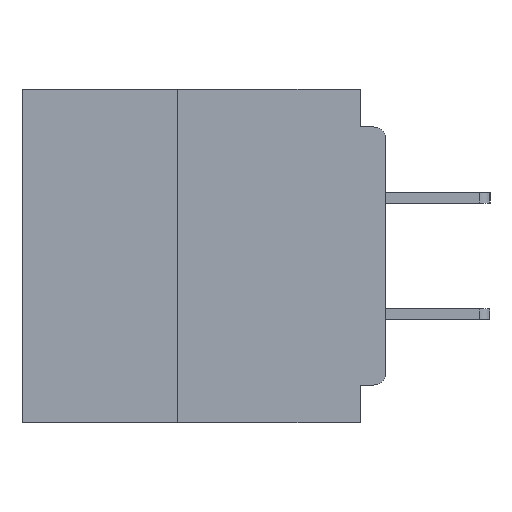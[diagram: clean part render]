
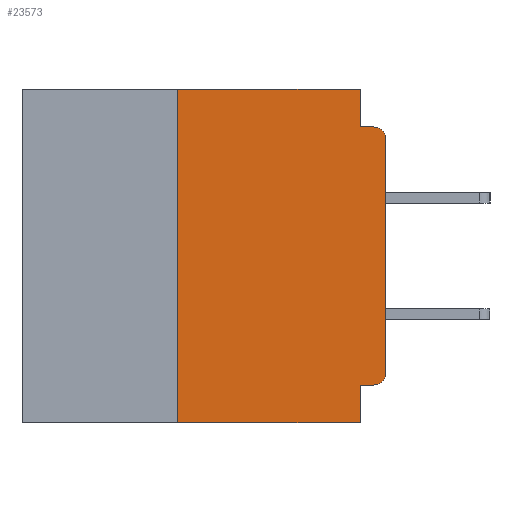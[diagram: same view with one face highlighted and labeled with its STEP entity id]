
A CAD part, left-side view. The second image highlights one B-rep face of the part: STEP entity #23573.
In plain terms, the highlighted planar face has unit normal (-1, 0, 0).
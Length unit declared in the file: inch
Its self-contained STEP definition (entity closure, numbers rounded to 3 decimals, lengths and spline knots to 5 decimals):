
#2146 = ORIENTED_EDGE ( 'NONE', *, *, #38937, .T. ) ;
#2557 = DIRECTION ( 'NONE',  ( 0., 0., 1. ) ) ;
#3601 = CARTESIAN_POINT ( 'NONE',  ( 0., 0.437, 0. ) ) ;
#5030 = EDGE_CURVE ( 'NONE', #21683, #59253, #38214, .T. ) ;
#5262 = DIRECTION ( 'NONE',  ( 0., -1., 0. ) ) ;
#6154 = CARTESIAN_POINT ( 'NONE',  ( 0., 0.015, -0.34 ) ) ;
#6610 = VECTOR ( 'NONE', #26562, 39.37008 ) ;
#6810 = CARTESIAN_POINT ( 'NONE',  ( 0., 0.25, 0. ) ) ;
#6912 = DIRECTION ( 'NONE',  ( 0., 0., -1. ) ) ;
#7923 = VECTOR ( 'NONE', #5262, 39.37008 ) ;
#8940 = DIRECTION ( 'NONE',  ( 0., 0., -1. ) ) ;
#8998 = LINE ( 'NONE', #47682, #6610 ) ;
#9124 = LINE ( 'NONE', #31560, #63652 ) ;
#9361 = ORIENTED_EDGE ( 'NONE', *, *, #5030, .F. ) ;
#9393 = VECTOR ( 'NONE', #68340, 39.37008 ) ;
#10102 = VECTOR ( 'NONE', #50333, 39.37008 ) ;
#10407 = CARTESIAN_POINT ( 'NONE',  ( 0., 0.25, -0.4 ) ) ;
#10498 = DIRECTION ( 'NONE',  ( 0., -1., 0. ) ) ;
#10693 = VERTEX_POINT ( 'NONE', #50213 ) ;
#11527 = DIRECTION ( 'NONE',  ( 0., 0., -1. ) ) ;
#11852 = ORIENTED_EDGE ( 'NONE', *, *, #23830, .F. ) ;
#12732 = LINE ( 'NONE', #10407, #9393 ) ;
#12925 = VECTOR ( 'NONE', #2557, 39.37008 ) ;
#14813 = EDGE_CURVE ( 'NONE', #66581, #22309, #45889, .T. ) ;
#15775 = CARTESIAN_POINT ( 'NONE',  ( 0., 0.015, -0.06 ) ) ;
#19424 = EDGE_CURVE ( 'NONE', #52553, #21683, #51793, .T. ) ;
#21014 = CARTESIAN_POINT ( 'NONE',  ( 0., 0., -0.34 ) ) ;
#21079 = DIRECTION ( 'NONE',  ( 0., 0., -1. ) ) ;
#21683 = VERTEX_POINT ( 'NONE', #24268 ) ;
#22309 = VERTEX_POINT ( 'NONE', #44845 ) ;
#22334 = FACE_OUTER_BOUND ( 'NONE', #32511, .T. ) ;
#22578 = ORIENTED_EDGE ( 'NONE', *, *, #50547, .F. ) ;
#23573 = ADVANCED_FACE ( 'NONE', ( #22334 ), #61561, .F. ) ;
#23830 = EDGE_CURVE ( 'NONE', #44612, #62760, #8998, .T. ) ;
#24268 = CARTESIAN_POINT ( 'NONE',  ( 0., 0.031, -0.355 ) ) ;
#24948 = EDGE_CURVE ( 'NONE', #22309, #52424, #61785, .T. ) ;
#26562 = DIRECTION ( 'NONE',  ( 0., -1., 0. ) ) ;
#27435 = AXIS2_PLACEMENT_3D ( 'NONE', #3601, #40567, #8940 ) ;
#27880 = ORIENTED_EDGE ( 'NONE', *, *, #38491, .F. ) ;
#28964 = CARTESIAN_POINT ( 'NONE',  ( 0., 0.031, -0.4 ) ) ;
#30287 = CARTESIAN_POINT ( 'NONE',  ( 0., 0.031, 0. ) ) ;
#30572 = CARTESIAN_POINT ( 'NONE',  ( 0., 0.015, -0.355 ) ) ;
#31560 = CARTESIAN_POINT ( 'NONE',  ( 0., 0., -0.045 ) ) ;
#32511 = EDGE_LOOP ( 'NONE', ( #47344, #59978, #64097, #27880, #11852, #22578, #2146, #9361, #41693, #43054 ) ) ;
#36944 = CARTESIAN_POINT ( 'NONE',  ( 0., 0.437, -0.4 ) ) ;
#38214 = LINE ( 'NONE', #45234, #10102 ) ;
#38491 = EDGE_CURVE ( 'NONE', #62760, #58154, #56256, .T. ) ;
#38937 = EDGE_CURVE ( 'NONE', #10693, #59253, #40485, .T. ) ;
#39795 = AXIS2_PLACEMENT_3D ( 'NONE', #15775, #52668, #21079 ) ;
#40485 = LINE ( 'NONE', #36944, #7923 ) ;
#40567 = DIRECTION ( 'NONE',  ( 1., 0., 0. ) ) ;
#41693 = ORIENTED_EDGE ( 'NONE', *, *, #19424, .F. ) ;
#42205 = VECTOR ( 'NONE', #6912, 39.37008 ) ;
#43054 = ORIENTED_EDGE ( 'NONE', *, *, #62907, .T. ) ;
#43089 = DIRECTION ( 'NONE',  ( -1., 0., 0. ) ) ;
#43285 = EDGE_CURVE ( 'NONE', #58154, #52424, #9124, .T. ) ;
#43556 = CIRCLE ( 'NONE', #66400, 0.015 ) ;
#43609 = CARTESIAN_POINT ( 'NONE',  ( 0., 0.031, 0. ) ) ;
#44612 = VERTEX_POINT ( 'NONE', #6810 ) ;
#44845 = CARTESIAN_POINT ( 'NONE',  ( 0., 0., -0.06 ) ) ;
#45234 = CARTESIAN_POINT ( 'NONE',  ( 0., 0.031, -0.4 ) ) ;
#45889 = LINE ( 'NONE', #50146, #12925 ) ;
#47344 = ORIENTED_EDGE ( 'NONE', *, *, #14813, .T. ) ;
#47439 = DIRECTION ( 'NONE',  ( 0., 1., 0. ) ) ;
#47682 = CARTESIAN_POINT ( 'NONE',  ( 0., 0.437, 0. ) ) ;
#50104 = VECTOR ( 'NONE', #47439, 39.37008 ) ;
#50146 = CARTESIAN_POINT ( 'NONE',  ( 0., 0., 0. ) ) ;
#50213 = CARTESIAN_POINT ( 'NONE',  ( 0., 0.25, -0.4 ) ) ;
#50333 = DIRECTION ( 'NONE',  ( 0., 0., -1. ) ) ;
#50547 = EDGE_CURVE ( 'NONE', #10693, #44612, #12732, .T. ) ;
#51793 = LINE ( 'NONE', #57868, #50104 ) ;
#52424 = VERTEX_POINT ( 'NONE', #61171 ) ;
#52553 = VERTEX_POINT ( 'NONE', #30572 ) ;
#52668 = DIRECTION ( 'NONE',  ( -1., 0., 0. ) ) ;
#56256 = LINE ( 'NONE', #43609, #42205 ) ;
#57868 = CARTESIAN_POINT ( 'NONE',  ( 0., 0., -0.355 ) ) ;
#58154 = VERTEX_POINT ( 'NONE', #61995 ) ;
#59253 = VERTEX_POINT ( 'NONE', #28964 ) ;
#59978 = ORIENTED_EDGE ( 'NONE', *, *, #24948, .T. ) ;
#61171 = CARTESIAN_POINT ( 'NONE',  ( 0., 0.015, -0.045 ) ) ;
#61561 = PLANE ( 'NONE',  #27435 ) ;
#61785 = CIRCLE ( 'NONE', #39795, 0.015 ) ;
#61995 = CARTESIAN_POINT ( 'NONE',  ( 0., 0.031, -0.045 ) ) ;
#62760 = VERTEX_POINT ( 'NONE', #30287 ) ;
#62907 = EDGE_CURVE ( 'NONE', #52553, #66581, #43556, .T. ) ;
#63652 = VECTOR ( 'NONE', #10498, 39.37008 ) ;
#64097 = ORIENTED_EDGE ( 'NONE', *, *, #43285, .F. ) ;
#66400 = AXIS2_PLACEMENT_3D ( 'NONE', #6154, #43089, #11527 ) ;
#66581 = VERTEX_POINT ( 'NONE', #21014 ) ;
#68340 = DIRECTION ( 'NONE',  ( 0., 0., 1. ) ) ;
